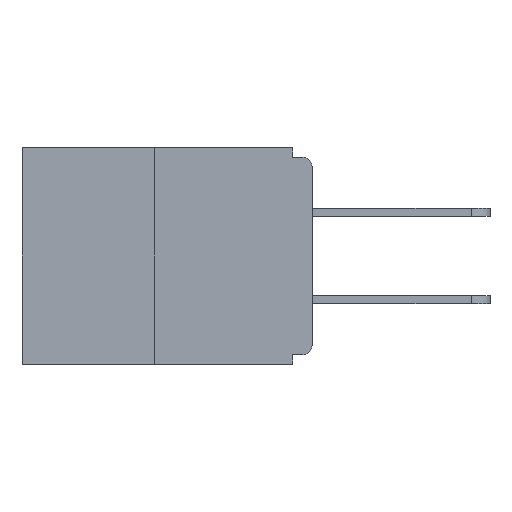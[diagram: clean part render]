
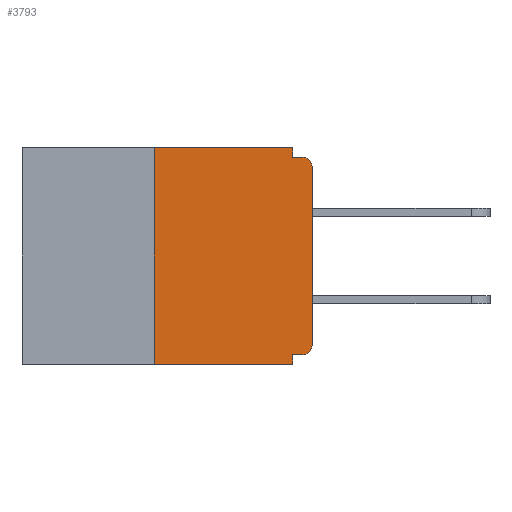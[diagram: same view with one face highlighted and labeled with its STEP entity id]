
A CAD part, left-side view. The second image highlights one B-rep face of the part: STEP entity #3793.
In plain terms, the highlighted planar face has unit normal (-1, 0, 0).
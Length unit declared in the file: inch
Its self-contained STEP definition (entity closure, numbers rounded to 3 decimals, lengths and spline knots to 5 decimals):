
#152 = CARTESIAN_POINT ( 'NONE',  ( 0., 0.25, 0. ) ) ;
#368 = ORIENTED_EDGE ( 'NONE', *, *, #8324, .T. ) ;
#724 = ORIENTED_EDGE ( 'NONE', *, *, #11133, .T. ) ;
#1151 = VECTOR ( 'NONE', #4083, 39.37008 ) ;
#1191 = ORIENTED_EDGE ( 'NONE', *, *, #17722, .T. ) ;
#1372 = VERTEX_POINT ( 'NONE', #10037 ) ;
#1467 = FACE_OUTER_BOUND ( 'NONE', #20934, .T. ) ;
#1532 = EDGE_CURVE ( 'NONE', #6881, #19176, #21718, .T. ) ;
#1770 = AXIS2_PLACEMENT_3D ( 'NONE', #12503, #5237, #7042 ) ;
#2068 = DIRECTION ( 'NONE',  ( -1., 0., 0. ) ) ;
#2127 = LINE ( 'NONE', #10794, #6419 ) ;
#2295 = DIRECTION ( 'NONE',  ( 1., 0., 0. ) ) ;
#2330 = CARTESIAN_POINT ( 'NONE',  ( 0., 0.031, 0. ) ) ;
#2700 = VECTOR ( 'NONE', #6998, 39.37008 ) ;
#3000 = EDGE_CURVE ( 'NONE', #14101, #1372, #13729, .T. ) ;
#3013 = VERTEX_POINT ( 'NONE', #12300 ) ;
#3287 = VERTEX_POINT ( 'NONE', #11962 ) ;
#3291 = LINE ( 'NONE', #6927, #2700 ) ;
#3562 = DIRECTION ( 'NONE',  ( 0., -1., 0. ) ) ;
#3711 = DIRECTION ( 'NONE',  ( 0., -1., 0. ) ) ;
#3793 = ADVANCED_FACE ( 'NONE', ( #1467 ), #14757, .F. ) ;
#3846 = CARTESIAN_POINT ( 'NONE',  ( 0., 0.015, -0.313 ) ) ;
#4083 = DIRECTION ( 'NONE',  ( 0., 0., 1. ) ) ;
#4365 = EDGE_CURVE ( 'NONE', #14412, #3013, #5720, .T. ) ;
#5237 = DIRECTION ( 'NONE',  ( -1., 0., 0. ) ) ;
#5543 = ORIENTED_EDGE ( 'NONE', *, *, #15145, .F. ) ;
#5720 = CIRCLE ( 'NONE', #1770, 0.015 ) ;
#5895 = CARTESIAN_POINT ( 'NONE',  ( 0., 0.46, 0. ) ) ;
#5972 = ORIENTED_EDGE ( 'NONE', *, *, #4365, .T. ) ;
#6317 = ORIENTED_EDGE ( 'NONE', *, *, #3000, .F. ) ;
#6419 = VECTOR ( 'NONE', #3711, 39.37008 ) ;
#6785 = EDGE_CURVE ( 'NONE', #21597, #17674, #10640, .T. ) ;
#6792 = AXIS2_PLACEMENT_3D ( 'NONE', #5895, #2295, #22102 ) ;
#6881 = VERTEX_POINT ( 'NONE', #18680 ) ;
#6927 = CARTESIAN_POINT ( 'NONE',  ( 0., 0.46, -0.343 ) ) ;
#6998 = DIRECTION ( 'NONE',  ( 0., -1., 0. ) ) ;
#7042 = DIRECTION ( 'NONE',  ( 0., 0., -1. ) ) ;
#7267 = LINE ( 'NONE', #16440, #9786 ) ;
#8324 = EDGE_CURVE ( 'NONE', #3287, #14412, #23065, .T. ) ;
#8874 = VECTOR ( 'NONE', #10760, 39.37008 ) ;
#9786 = VECTOR ( 'NONE', #3562, 39.37008 ) ;
#10037 = CARTESIAN_POINT ( 'NONE',  ( 0., 0.031, -0.343 ) ) ;
#10640 = LINE ( 'NONE', #152, #15510 ) ;
#10760 = DIRECTION ( 'NONE',  ( 0., 0., -1. ) ) ;
#10761 = ORIENTED_EDGE ( 'NONE', *, *, #22198, .F. ) ;
#10794 = CARTESIAN_POINT ( 'NONE',  ( 0., 0.46, 0. ) ) ;
#10910 = CARTESIAN_POINT ( 'NONE',  ( 0., 0.25, 0. ) ) ;
#11133 = EDGE_CURVE ( 'NONE', #21597, #1372, #3291, .T. ) ;
#11827 = ORIENTED_EDGE ( 'NONE', *, *, #21403, .F. ) ;
#11962 = CARTESIAN_POINT ( 'NONE',  ( 0., 0., -0.313 ) ) ;
#12300 = CARTESIAN_POINT ( 'NONE',  ( 0., 0.015, -0.015 ) ) ;
#12432 = CIRCLE ( 'NONE', #22237, 0.015 ) ;
#12503 = CARTESIAN_POINT ( 'NONE',  ( 0., 0.015, -0.03 ) ) ;
#12629 = DIRECTION ( 'NONE',  ( 0., 0., -1. ) ) ;
#12686 = DIRECTION ( 'NONE',  ( 0., 1., 0. ) ) ;
#12756 = VERTEX_POINT ( 'NONE', #20894 ) ;
#12809 = LINE ( 'NONE', #23556, #23391 ) ;
#13729 = LINE ( 'NONE', #22780, #8874 ) ;
#14101 = VERTEX_POINT ( 'NONE', #18542 ) ;
#14412 = VERTEX_POINT ( 'NONE', #20489 ) ;
#14757 = PLANE ( 'NONE',  #6792 ) ;
#15145 = EDGE_CURVE ( 'NONE', #12756, #14101, #12809, .T. ) ;
#15510 = VECTOR ( 'NONE', #19888, 39.37008 ) ;
#16440 = CARTESIAN_POINT ( 'NONE',  ( 0., 0., -0.015 ) ) ;
#17674 = VERTEX_POINT ( 'NONE', #10910 ) ;
#17722 = EDGE_CURVE ( 'NONE', #12756, #3287, #12432, .T. ) ;
#18299 = CARTESIAN_POINT ( 'NONE',  ( 0., 0., 0. ) ) ;
#18542 = CARTESIAN_POINT ( 'NONE',  ( 0., 0.031, -0.328 ) ) ;
#18680 = CARTESIAN_POINT ( 'NONE',  ( 0., 0.031, 0. ) ) ;
#19176 = VERTEX_POINT ( 'NONE', #20031 ) ;
#19888 = DIRECTION ( 'NONE',  ( 0., 0., 1. ) ) ;
#20024 = ORIENTED_EDGE ( 'NONE', *, *, #1532, .F. ) ;
#20031 = CARTESIAN_POINT ( 'NONE',  ( 0., 0.031, -0.015 ) ) ;
#20169 = DIRECTION ( 'NONE',  ( 0., 0., -1. ) ) ;
#20489 = CARTESIAN_POINT ( 'NONE',  ( 0., 0., -0.03 ) ) ;
#20615 = CARTESIAN_POINT ( 'NONE',  ( 0., 0.25, -0.343 ) ) ;
#20894 = CARTESIAN_POINT ( 'NONE',  ( 0., 0.015, -0.328 ) ) ;
#20934 = EDGE_LOOP ( 'NONE', ( #10761, #23189, #724, #6317, #5543, #1191, #368, #5972, #11827, #20024 ) ) ;
#21136 = VECTOR ( 'NONE', #20169, 39.37008 ) ;
#21403 = EDGE_CURVE ( 'NONE', #19176, #3013, #7267, .T. ) ;
#21597 = VERTEX_POINT ( 'NONE', #20615 ) ;
#21718 = LINE ( 'NONE', #2330, #21136 ) ;
#22102 = DIRECTION ( 'NONE',  ( 0., 0., -1. ) ) ;
#22198 = EDGE_CURVE ( 'NONE', #17674, #6881, #2127, .T. ) ;
#22237 = AXIS2_PLACEMENT_3D ( 'NONE', #3846, #2068, #12629 ) ;
#22780 = CARTESIAN_POINT ( 'NONE',  ( 0., 0.031, -0.343 ) ) ;
#23065 = LINE ( 'NONE', #18299, #1151 ) ;
#23189 = ORIENTED_EDGE ( 'NONE', *, *, #6785, .F. ) ;
#23391 = VECTOR ( 'NONE', #12686, 39.37008 ) ;
#23556 = CARTESIAN_POINT ( 'NONE',  ( 0., 0., -0.328 ) ) ;
